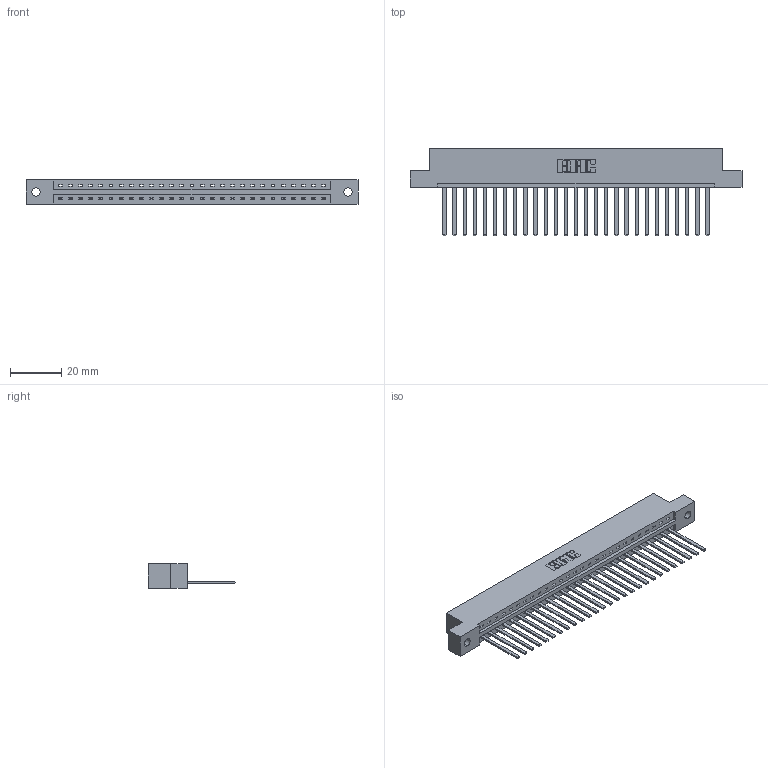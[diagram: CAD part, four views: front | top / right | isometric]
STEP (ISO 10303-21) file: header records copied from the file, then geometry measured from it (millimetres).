
FILE_DESCRIPTION (( 'STEP AP203' ), '1' );
FILE_NAME ('337-027-544-102.STEP', '2018-08-06T08:15:26', ( '' ), ( '' ), 'SwSTEP 2.0', 'SolidWorks 2016', '' );
FILE_SCHEMA (( 'CONFIG_CONTROL_DESIGN' ));
Length unit declared in the file: inch
Products named in the file (3): 337 Part_Flush Mounting Lugs - 0.128 Dia; 345-292-001_345-293-144; 337-027-544-102
Assembly tree (28 placements, depth 2):
  337-027-544-102
    337 Part_Flush Mounting Lugs - 0.128 Dia
    345-292-001_345-293-144  x27
Bounding box: 130 x 34.3 x 9.4 mm (x, y, z)
Volume: 13599.3 mm3; surface area: 14728.4 mm2
Topology: 28 solids, 28 shells, 1626 faces, 4901 edges, 3230 vertices
Faces by surface type: plane 1204, cylinder 422
Entity records: 21829 total; most frequent: CARTESIAN_POINT 3807, ORIENTED_EDGE 3770, DIRECTION 3231, EDGE_CURVE 1885, VECTOR 1761, LINE 1761, VERTEX_POINT 1254, AXIS2_PLACEMENT_3D 735
